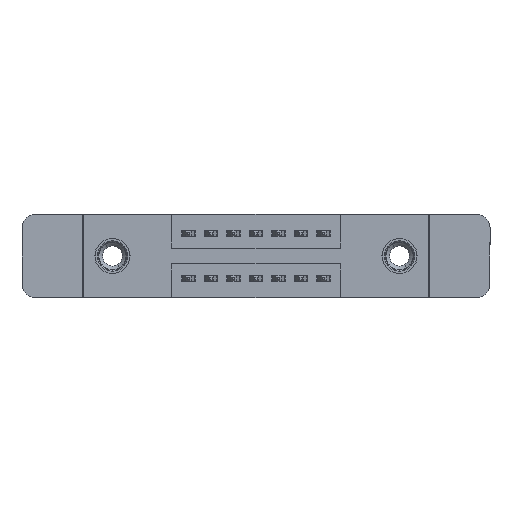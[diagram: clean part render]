
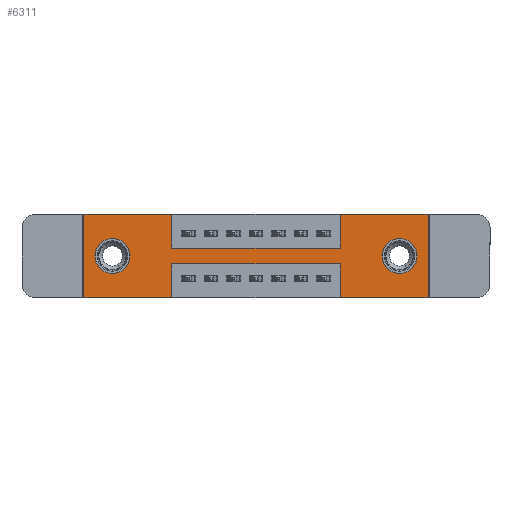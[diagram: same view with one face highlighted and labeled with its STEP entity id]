
A CAD part, front view. The second image highlights one B-rep face of the part: STEP entity #6311.
In plain terms, the highlighted planar face has unit normal (0, -1, 0).
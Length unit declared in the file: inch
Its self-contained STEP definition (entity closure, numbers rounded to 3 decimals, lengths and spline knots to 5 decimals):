
#83 = CARTESIAN_POINT ( 'NONE',  ( 1.1425, 0., -0.37 ) ) ;
#84 = EDGE_CURVE ( 'NONE', #2582, #14690, #11344, .T. ) ;
#181 = EDGE_CURVE ( 'NONE', #10015, #8504, #6738, .T. ) ;
#659 = CARTESIAN_POINT ( 'NONE',  ( 1.405, 0., -0.107 ) ) ;
#685 = CARTESIAN_POINT ( 'NONE',  ( 0., 0., 0. ) ) ;
#997 = LINE ( 'NONE', #4990, #13299 ) ;
#1076 = ORIENTED_EDGE ( 'NONE', *, *, #181, .F. ) ;
#1098 = CARTESIAN_POINT ( 'NONE',  ( 0.3925, 0., -0.37 ) ) ;
#1124 = EDGE_CURVE ( 'NONE', #2659, #14390, #7314, .T. ) ;
#1266 = LINE ( 'NONE', #1919, #7630 ) ;
#1738 = CARTESIAN_POINT ( 'NONE',  ( 0., 0., 0. ) ) ;
#1752 = CARTESIAN_POINT ( 'NONE',  ( 0.13, 0., -0.185 ) ) ;
#1884 = ORIENTED_EDGE ( 'NONE', *, *, #11931, .T. ) ;
#1887 = DIRECTION ( 'NONE',  ( 1., 0., 0. ) ) ;
#1905 = DIRECTION ( 'NONE',  ( 0., 1., 0. ) ) ;
#1919 = CARTESIAN_POINT ( 'NONE',  ( 0.3925, 0., -0.22 ) ) ;
#1987 = CARTESIAN_POINT ( 'NONE',  ( 1.535, 0., 0. ) ) ;
#2015 = CIRCLE ( 'NONE', #13051, 0.078 ) ;
#2210 = ORIENTED_EDGE ( 'NONE', *, *, #14314, .T. ) ;
#2235 = DIRECTION ( 'NONE',  ( -1., 0., 0. ) ) ;
#2332 = ORIENTED_EDGE ( 'NONE', *, *, #8784, .F. ) ;
#2365 = CARTESIAN_POINT ( 'NONE',  ( 1.405, 0., -0.263 ) ) ;
#2582 = VERTEX_POINT ( 'NONE', #7442 ) ;
#2659 = VERTEX_POINT ( 'NONE', #2365 ) ;
#2679 = AXIS2_PLACEMENT_3D ( 'NONE', #14526, #6297, #14581 ) ;
#2733 = LINE ( 'NONE', #9007, #5927 ) ;
#2796 = VECTOR ( 'NONE', #2235, 39.37008 ) ;
#2916 = VECTOR ( 'NONE', #12185, 39.37008 ) ;
#2967 = DIRECTION ( 'NONE',  ( 1., 0., 0. ) ) ;
#2981 = DIRECTION ( 'NONE',  ( 0., 0., 1. ) ) ;
#3138 = EDGE_CURVE ( 'NONE', #11777, #10239, #6725, .T. ) ;
#3234 = ORIENTED_EDGE ( 'NONE', *, *, #9643, .F. ) ;
#3625 = VERTEX_POINT ( 'NONE', #1098 ) ;
#3974 = ORIENTED_EDGE ( 'NONE', *, *, #13575, .F. ) ;
#4283 = ORIENTED_EDGE ( 'NONE', *, *, #10780, .F. ) ;
#4312 = CARTESIAN_POINT ( 'NONE',  ( 0.3925, 0., -0.15 ) ) ;
#4375 = DIRECTION ( 'NONE',  ( 0., 1., 0. ) ) ;
#4412 = FACE_BOUND ( 'NONE', #12129, .T. ) ;
#4603 = EDGE_CURVE ( 'NONE', #14390, #2659, #4655, .T. ) ;
#4655 = CIRCLE ( 'NONE', #7662, 0.078 ) ;
#4990 = CARTESIAN_POINT ( 'NONE',  ( 0.3925, 0., -0.37 ) ) ;
#5017 = ORIENTED_EDGE ( 'NONE', *, *, #1124, .T. ) ;
#5225 = EDGE_CURVE ( 'NONE', #12413, #9599, #2733, .T. ) ;
#5465 = DIRECTION ( 'NONE',  ( 0., 0., 1. ) ) ;
#5536 = CARTESIAN_POINT ( 'NONE',  ( 1.1425, 0., 0. ) ) ;
#5589 = DIRECTION ( 'NONE',  ( 0., 0., -1. ) ) ;
#5594 = ORIENTED_EDGE ( 'NONE', *, *, #7082, .F. ) ;
#5597 = CARTESIAN_POINT ( 'NONE',  ( 0., 0., 0. ) ) ;
#5796 = DIRECTION ( 'NONE',  ( -1., 0., 0. ) ) ;
#5821 = VECTOR ( 'NONE', #5796, 39.37008 ) ;
#5927 = VECTOR ( 'NONE', #12572, 39.37008 ) ;
#5991 = LINE ( 'NONE', #8182, #2796 ) ;
#6229 = LINE ( 'NONE', #1738, #11778 ) ;
#6246 = VERTEX_POINT ( 'NONE', #12100 ) ;
#6297 = DIRECTION ( 'NONE',  ( 0., -1., 0. ) ) ;
#6311 = ADVANCED_FACE ( 'NONE', ( #10311, #4412, #13874 ), #13428, .T. ) ;
#6547 = CARTESIAN_POINT ( 'NONE',  ( 0.13, 0., -0.107 ) ) ;
#6654 = AXIS2_PLACEMENT_3D ( 'NONE', #11664, #11660, #11644 ) ;
#6725 = LINE ( 'NONE', #5597, #15401 ) ;
#6738 = LINE ( 'NONE', #14708, #9843 ) ;
#6771 = VERTEX_POINT ( 'NONE', #12567 ) ;
#6846 = VERTEX_POINT ( 'NONE', #1987 ) ;
#6941 = LINE ( 'NONE', #685, #9684 ) ;
#7082 = EDGE_CURVE ( 'NONE', #6246, #3625, #997, .T. ) ;
#7313 = CARTESIAN_POINT ( 'NONE',  ( 1.1425, 0., -0.15 ) ) ;
#7314 = CIRCLE ( 'NONE', #6654, 0.078 ) ;
#7341 = EDGE_LOOP ( 'NONE', ( #5594, #14521, #3974, #14693, #3234, #7931, #7531, #2332, #1076, #9932, #13005, #4283 ) ) ;
#7442 = CARTESIAN_POINT ( 'NONE',  ( 1.535, 0., -0.37 ) ) ;
#7531 = ORIENTED_EDGE ( 'NONE', *, *, #5225, .F. ) ;
#7630 = VECTOR ( 'NONE', #12658, 39.37008 ) ;
#7662 = AXIS2_PLACEMENT_3D ( 'NONE', #9023, #1905, #10216 ) ;
#7912 = EDGE_CURVE ( 'NONE', #10239, #10015, #6229, .T. ) ;
#7931 = ORIENTED_EDGE ( 'NONE', *, *, #10066, .F. ) ;
#7956 = CARTESIAN_POINT ( 'NONE',  ( 1.535, 0., 0. ) ) ;
#8182 = CARTESIAN_POINT ( 'NONE',  ( 0., 0., -0.37 ) ) ;
#8290 = CARTESIAN_POINT ( 'NONE',  ( 0.3925, 0., -0.15 ) ) ;
#8504 = VERTEX_POINT ( 'NONE', #4312 ) ;
#8558 = AXIS2_PLACEMENT_3D ( 'NONE', #1752, #10068, #2981 ) ;
#8592 = DIRECTION ( 'NONE',  ( 0., 0., -1. ) ) ;
#8784 = EDGE_CURVE ( 'NONE', #8504, #12413, #10287, .T. ) ;
#9007 = CARTESIAN_POINT ( 'NONE',  ( 1.1425, 0., 0. ) ) ;
#9023 = CARTESIAN_POINT ( 'NONE',  ( 1.405, 0., -0.185 ) ) ;
#9599 = VERTEX_POINT ( 'NONE', #5536 ) ;
#9643 = EDGE_CURVE ( 'NONE', #6846, #2582, #12133, .T. ) ;
#9684 = VECTOR ( 'NONE', #1887, 39.37008 ) ;
#9843 = VECTOR ( 'NONE', #10013, 39.37008 ) ;
#9901 = VECTOR ( 'NONE', #14197, 39.37008 ) ;
#9932 = ORIENTED_EDGE ( 'NONE', *, *, #7912, .F. ) ;
#10013 = DIRECTION ( 'NONE',  ( 0., 0., -1. ) ) ;
#10015 = VERTEX_POINT ( 'NONE', #13663 ) ;
#10017 = VERTEX_POINT ( 'NONE', #6547 ) ;
#10066 = EDGE_CURVE ( 'NONE', #9599, #6846, #6941, .T. ) ;
#10068 = DIRECTION ( 'NONE',  ( 0., 1., 0. ) ) ;
#10216 = DIRECTION ( 'NONE',  ( 0., 0., -1. ) ) ;
#10239 = VERTEX_POINT ( 'NONE', #10447 ) ;
#10287 = LINE ( 'NONE', #8290, #9901 ) ;
#10311 = FACE_BOUND ( 'NONE', #13964, .T. ) ;
#10447 = CARTESIAN_POINT ( 'NONE',  ( 0., 0., 0. ) ) ;
#10780 = EDGE_CURVE ( 'NONE', #3625, #11777, #5991, .T. ) ;
#11127 = CARTESIAN_POINT ( 'NONE',  ( 0., 0., -0.37 ) ) ;
#11344 = LINE ( 'NONE', #15279, #5821 ) ;
#11452 = CARTESIAN_POINT ( 'NONE',  ( 0.13, 0., -0.185 ) ) ;
#11644 = DIRECTION ( 'NONE',  ( 0., 0., -1. ) ) ;
#11660 = DIRECTION ( 'NONE',  ( 0., 1., 0. ) ) ;
#11664 = CARTESIAN_POINT ( 'NONE',  ( 1.405, 0., -0.185 ) ) ;
#11777 = VERTEX_POINT ( 'NONE', #11127 ) ;
#11778 = VECTOR ( 'NONE', #2967, 39.37008 ) ;
#11931 = EDGE_CURVE ( 'NONE', #6771, #10017, #2015, .T. ) ;
#12100 = CARTESIAN_POINT ( 'NONE',  ( 0.3925, 0., -0.22 ) ) ;
#12129 = EDGE_LOOP ( 'NONE', ( #2210, #1884 ) ) ;
#12133 = LINE ( 'NONE', #7956, #14904 ) ;
#12185 = DIRECTION ( 'NONE',  ( 0., 0., 1. ) ) ;
#12248 = CARTESIAN_POINT ( 'NONE',  ( 1.1425, 0., -0.37 ) ) ;
#12413 = VERTEX_POINT ( 'NONE', #7313 ) ;
#12567 = CARTESIAN_POINT ( 'NONE',  ( 0.13, 0., -0.263 ) ) ;
#12572 = DIRECTION ( 'NONE',  ( 0., 0., 1. ) ) ;
#12631 = CARTESIAN_POINT ( 'NONE',  ( 1.1425, 0., -0.22 ) ) ;
#12658 = DIRECTION ( 'NONE',  ( -1., 0., 0. ) ) ;
#12685 = DIRECTION ( 'NONE',  ( 0., 0., 1. ) ) ;
#13005 = ORIENTED_EDGE ( 'NONE', *, *, #3138, .F. ) ;
#13051 = AXIS2_PLACEMENT_3D ( 'NONE', #11452, #4375, #12685 ) ;
#13299 = VECTOR ( 'NONE', #8592, 39.37008 ) ;
#13428 = PLANE ( 'NONE',  #2679 ) ;
#13575 = EDGE_CURVE ( 'NONE', #14690, #14802, #15161, .T. ) ;
#13663 = CARTESIAN_POINT ( 'NONE',  ( 0.3925, 0., 0. ) ) ;
#13874 = FACE_OUTER_BOUND ( 'NONE', #7341, .T. ) ;
#13964 = EDGE_LOOP ( 'NONE', ( #14963, #5017 ) ) ;
#14197 = DIRECTION ( 'NONE',  ( 1., 0., 0. ) ) ;
#14314 = EDGE_CURVE ( 'NONE', #10017, #6771, #15039, .T. ) ;
#14390 = VERTEX_POINT ( 'NONE', #659 ) ;
#14426 = EDGE_CURVE ( 'NONE', #14802, #6246, #1266, .T. ) ;
#14521 = ORIENTED_EDGE ( 'NONE', *, *, #14426, .F. ) ;
#14526 = CARTESIAN_POINT ( 'NONE',  ( 0., 0., -0.37 ) ) ;
#14581 = DIRECTION ( 'NONE',  ( 0., 0., -1. ) ) ;
#14690 = VERTEX_POINT ( 'NONE', #12248 ) ;
#14693 = ORIENTED_EDGE ( 'NONE', *, *, #84, .F. ) ;
#14708 = CARTESIAN_POINT ( 'NONE',  ( 0.3925, 0., 0. ) ) ;
#14802 = VERTEX_POINT ( 'NONE', #12631 ) ;
#14904 = VECTOR ( 'NONE', #5589, 39.37008 ) ;
#14963 = ORIENTED_EDGE ( 'NONE', *, *, #4603, .T. ) ;
#15039 = CIRCLE ( 'NONE', #8558, 0.078 ) ;
#15161 = LINE ( 'NONE', #83, #2916 ) ;
#15279 = CARTESIAN_POINT ( 'NONE',  ( 0., 0., -0.37 ) ) ;
#15401 = VECTOR ( 'NONE', #5465, 39.37008 ) ;
